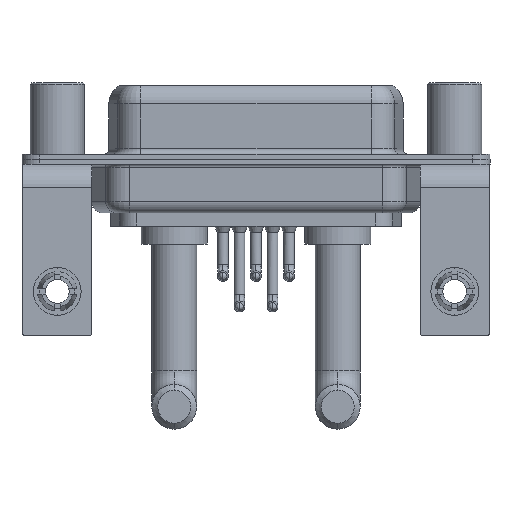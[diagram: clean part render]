
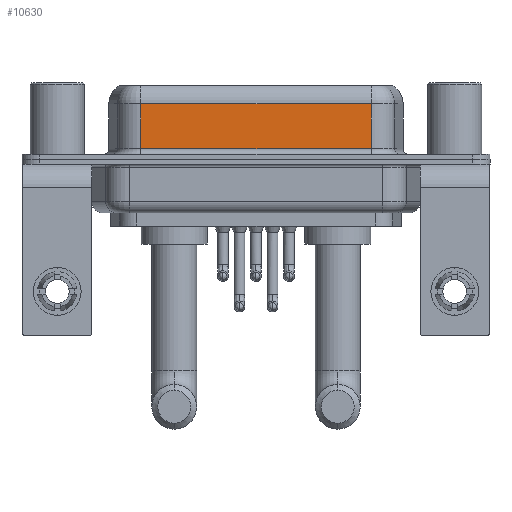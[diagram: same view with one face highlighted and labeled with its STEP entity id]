
A CAD part, front view. The second image highlights one B-rep face of the part: STEP entity #10630.
In plain terms, the highlighted planar face has unit normal (0, -1, 0).
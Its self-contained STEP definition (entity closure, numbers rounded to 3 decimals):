
#487 = ORIENTED_EDGE ( 'NONE', *, *, #6862, .T. ) ;
#583 = EDGE_LOOP ( 'NONE', ( #8214, #11066, #487, #15998 ) ) ;
#610 = VECTOR ( 'NONE', #3283, 1000. ) ;
#1806 = EDGE_CURVE ( 'NONE', #3286, #14418, #11748, .T. ) ;
#2632 = CARTESIAN_POINT ( 'NONE',  ( 7.013, -3.95, 4.65 ) ) ;
#3283 = DIRECTION ( 'NONE',  ( 0., 0., -1. ) ) ;
#3286 = VERTEX_POINT ( 'NONE', #9186 ) ;
#3800 = DIRECTION ( 'NONE',  ( 1., 0., 0. ) ) ;
#4264 = DIRECTION ( 'NONE',  ( 0., 1., 0. ) ) ;
#4365 = DIRECTION ( 'NONE',  ( 0., 0., 1. ) ) ;
#6288 = VECTOR ( 'NONE', #14028, 1000. ) ;
#6862 = EDGE_CURVE ( 'NONE', #14418, #11407, #17663, .T. ) ;
#7296 = EDGE_CURVE ( 'NONE', #3286, #16212, #17322, .T. ) ;
#8214 = ORIENTED_EDGE ( 'NONE', *, *, #7296, .F. ) ;
#9186 = CARTESIAN_POINT ( 'NONE',  ( 26.287, -3.95, 4.65 ) ) ;
#10630 = ADVANCED_FACE ( 'NONE', ( #12218 ), #18430, .F. ) ;
#11066 = ORIENTED_EDGE ( 'NONE', *, *, #1806, .T. ) ;
#11407 = VERTEX_POINT ( 'NONE', #13230 ) ;
#11748 = LINE ( 'NONE', #18266, #15654 ) ;
#12218 = FACE_OUTER_BOUND ( 'NONE', #583, .T. ) ;
#13230 = CARTESIAN_POINT ( 'NONE',  ( 7.013, -3.95, 0.9 ) ) ;
#13613 = DIRECTION ( 'NONE',  ( -1., 0., 0. ) ) ;
#13965 = CARTESIAN_POINT ( 'NONE',  ( 26.287, -3.95, 0.9 ) ) ;
#14028 = DIRECTION ( 'NONE',  ( 0., 0., -1. ) ) ;
#14113 = CARTESIAN_POINT ( 'NONE',  ( 26.287, -3.95, 6.4 ) ) ;
#14418 = VERTEX_POINT ( 'NONE', #2632 ) ;
#15585 = CARTESIAN_POINT ( 'NONE',  ( 7.013, -3.95, 6.4 ) ) ;
#15654 = VECTOR ( 'NONE', #13613, 1000. ) ;
#15724 = EDGE_CURVE ( 'NONE', #11407, #16212, #16404, .T. ) ;
#15998 = ORIENTED_EDGE ( 'NONE', *, *, #15724, .T. ) ;
#16212 = VERTEX_POINT ( 'NONE', #13965 ) ;
#16299 = AXIS2_PLACEMENT_3D ( 'NONE', #18537, #4264, #4365 ) ;
#16404 = LINE ( 'NONE', #19322, #17767 ) ;
#17322 = LINE ( 'NONE', #14113, #610 ) ;
#17663 = LINE ( 'NONE', #15585, #6288 ) ;
#17767 = VECTOR ( 'NONE', #3800, 1000. ) ;
#18266 = CARTESIAN_POINT ( 'NONE',  ( 26.287, -3.95, 4.65 ) ) ;
#18430 = PLANE ( 'NONE',  #16299 ) ;
#18537 = CARTESIAN_POINT ( 'NONE',  ( 26.287, -3.95, 6.4 ) ) ;
#19322 = CARTESIAN_POINT ( 'NONE',  ( 26.287, -3.95, 0.9 ) ) ;
